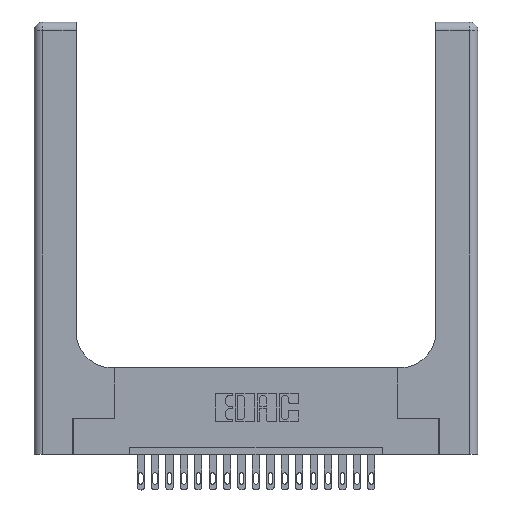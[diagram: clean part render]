
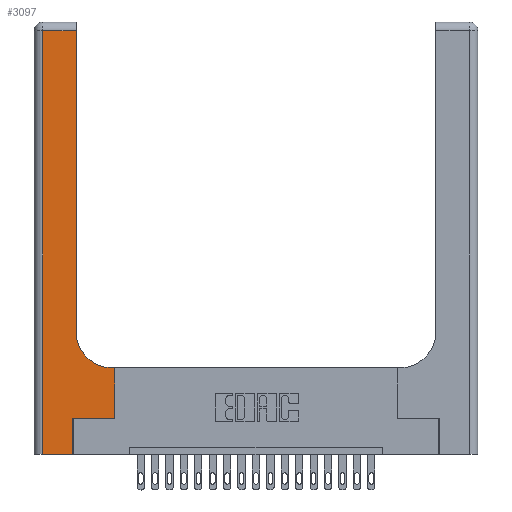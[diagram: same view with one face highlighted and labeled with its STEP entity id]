
A CAD part, top view. The second image highlights one B-rep face of the part: STEP entity #3097.
In plain terms, the highlighted planar face has unit normal (0, 0, 1).
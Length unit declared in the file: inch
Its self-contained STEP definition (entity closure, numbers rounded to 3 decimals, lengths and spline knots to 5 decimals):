
#13 = DIRECTION ( 'NONE',  ( -1., 0., 0. ) ) ;
#112 = DIRECTION ( 'NONE',  ( 0., 1., 0. ) ) ;
#179 = CARTESIAN_POINT ( 'NONE',  ( 0.2915, 0.6, 0.37 ) ) ;
#181 = ORIENTED_EDGE ( 'NONE', *, *, #9121, .T. ) ;
#275 = VERTEX_POINT ( 'NONE', #9703 ) ;
#402 = EDGE_LOOP ( 'NONE', ( #1958, #13877, #4231, #14845, #14427, #1934, #3012, #6285, #181 ) ) ;
#1058 = EDGE_CURVE ( 'NONE', #4562, #6949, #6552, .T. ) ;
#1400 = CIRCLE ( 'NONE', #17150, 0.25 ) ;
#1844 = CARTESIAN_POINT ( 'NONE',  ( 0., 3., 0.37 ) ) ;
#1934 = ORIENTED_EDGE ( 'NONE', *, *, #6900, .T. ) ;
#1958 = ORIENTED_EDGE ( 'NONE', *, *, #1058, .T. ) ;
#2052 = VECTOR ( 'NONE', #6782, 39.37008 ) ;
#3012 = ORIENTED_EDGE ( 'NONE', *, *, #17162, .T. ) ;
#3097 = ADVANCED_FACE ( 'NONE', ( #14431 ), #11414, .F. ) ;
#3114 = VERTEX_POINT ( 'NONE', #11489 ) ;
#3154 = EDGE_CURVE ( 'NONE', #3114, #15328, #4426, .T. ) ;
#3276 = EDGE_CURVE ( 'NONE', #275, #3114, #17510, .T. ) ;
#3555 = DIRECTION ( 'NONE',  ( 0., 0., -1. ) ) ;
#3893 = VERTEX_POINT ( 'NONE', #13837 ) ;
#3973 = LINE ( 'NONE', #16396, #4221 ) ;
#4108 = CARTESIAN_POINT ( 'NONE',  ( 0.269, 0.25, 0.37 ) ) ;
#4221 = VECTOR ( 'NONE', #4911, 39.37008 ) ;
#4231 = ORIENTED_EDGE ( 'NONE', *, *, #19730, .T. ) ;
#4426 = LINE ( 'NONE', #19972, #19048 ) ;
#4562 = VERTEX_POINT ( 'NONE', #20212 ) ;
#4911 = DIRECTION ( 'NONE',  ( -1., 0., 0. ) ) ;
#5025 = EDGE_CURVE ( 'NONE', #3893, #14383, #5359, .T. ) ;
#5359 = LINE ( 'NONE', #179, #2052 ) ;
#5488 = CARTESIAN_POINT ( 'NONE',  ( 0.5415, 0.6, 0.37 ) ) ;
#5720 = CARTESIAN_POINT ( 'NONE',  ( 0.2915, 2.94, 0.37 ) ) ;
#5948 = CARTESIAN_POINT ( 'NONE',  ( 0.269, 0.25, 0.37 ) ) ;
#6042 = VECTOR ( 'NONE', #19911, 39.37008 ) ;
#6081 = DIRECTION ( 'NONE',  ( 0., -1., 0. ) ) ;
#6092 = LINE ( 'NONE', #4108, #15083 ) ;
#6285 = ORIENTED_EDGE ( 'NONE', *, *, #5025, .T. ) ;
#6552 = LINE ( 'NONE', #8650, #6042 ) ;
#6782 = DIRECTION ( 'NONE',  ( -1., 0., 0. ) ) ;
#6900 = EDGE_CURVE ( 'NONE', #15328, #10417, #6092, .T. ) ;
#6949 = VERTEX_POINT ( 'NONE', #5720 ) ;
#7441 = CARTESIAN_POINT ( 'NONE',  ( 0.5415, 0.85, 0.37 ) ) ;
#7669 = CARTESIAN_POINT ( 'NONE',  ( 0.06, 3., 0.37 ) ) ;
#8154 = LINE ( 'NONE', #11465, #15090 ) ;
#8160 = CARTESIAN_POINT ( 'NONE',  ( 0., 0., 0.37 ) ) ;
#8528 = LINE ( 'NONE', #7669, #11089 ) ;
#8532 = VECTOR ( 'NONE', #13289, 39.37008 ) ;
#8650 = CARTESIAN_POINT ( 'NONE',  ( 0.2915, 3., 0.37 ) ) ;
#9090 = DIRECTION ( 'NONE',  ( 1., 0., 0. ) ) ;
#9121 = EDGE_CURVE ( 'NONE', #14383, #4562, #1400, .T. ) ;
#9625 = DIRECTION ( 'NONE',  ( 0., 1., 0. ) ) ;
#9703 = CARTESIAN_POINT ( 'NONE',  ( 0.06, 0., 0.37 ) ) ;
#10417 = VERTEX_POINT ( 'NONE', #12337 ) ;
#11089 = VECTOR ( 'NONE', #6081, 39.37008 ) ;
#11414 = PLANE ( 'NONE',  #14020 ) ;
#11465 = CARTESIAN_POINT ( 'NONE',  ( 0.5585, 0.25, 0.37 ) ) ;
#11489 = CARTESIAN_POINT ( 'NONE',  ( 0.269, 0., 0.37 ) ) ;
#11580 = CARTESIAN_POINT ( 'NONE',  ( 0.06, 2.94, 0.37 ) ) ;
#12337 = CARTESIAN_POINT ( 'NONE',  ( 0.5585, 0.25, 0.37 ) ) ;
#12361 = DIRECTION ( 'NONE',  ( 0., 0., -1. ) ) ;
#12943 = EDGE_CURVE ( 'NONE', #6949, #14182, #3973, .T. ) ;
#13289 = DIRECTION ( 'NONE',  ( 1., 0., 0. ) ) ;
#13837 = CARTESIAN_POINT ( 'NONE',  ( 0.5585, 0.6, 0.37 ) ) ;
#13877 = ORIENTED_EDGE ( 'NONE', *, *, #12943, .T. ) ;
#13908 = DIRECTION ( 'NONE',  ( 1., 0., 0. ) ) ;
#14020 = AXIS2_PLACEMENT_3D ( 'NONE', #1844, #3555, #13 ) ;
#14182 = VERTEX_POINT ( 'NONE', #11580 ) ;
#14383 = VERTEX_POINT ( 'NONE', #5488 ) ;
#14427 = ORIENTED_EDGE ( 'NONE', *, *, #3154, .T. ) ;
#14431 = FACE_OUTER_BOUND ( 'NONE', #402, .T. ) ;
#14845 = ORIENTED_EDGE ( 'NONE', *, *, #3276, .T. ) ;
#15083 = VECTOR ( 'NONE', #13908, 39.37008 ) ;
#15090 = VECTOR ( 'NONE', #9625, 39.37008 ) ;
#15328 = VERTEX_POINT ( 'NONE', #5948 ) ;
#16396 = CARTESIAN_POINT ( 'NONE',  ( 0., 2.94, 0.37 ) ) ;
#17150 = AXIS2_PLACEMENT_3D ( 'NONE', #7441, #12361, #9090 ) ;
#17162 = EDGE_CURVE ( 'NONE', #10417, #3893, #8154, .T. ) ;
#17510 = LINE ( 'NONE', #8160, #8532 ) ;
#19048 = VECTOR ( 'NONE', #112, 39.37008 ) ;
#19730 = EDGE_CURVE ( 'NONE', #14182, #275, #8528, .T. ) ;
#19911 = DIRECTION ( 'NONE',  ( 0., 1., 0. ) ) ;
#19972 = CARTESIAN_POINT ( 'NONE',  ( 0.269, 0., 0.37 ) ) ;
#20212 = CARTESIAN_POINT ( 'NONE',  ( 0.2915, 0.85, 0.37 ) ) ;
